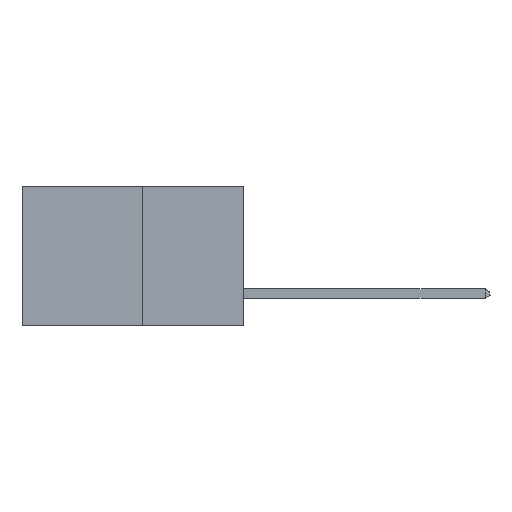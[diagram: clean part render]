
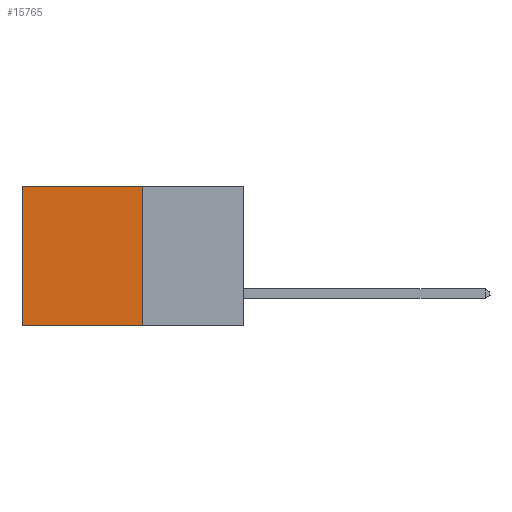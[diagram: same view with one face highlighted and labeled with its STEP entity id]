
A CAD part, left-side view. The second image highlights one B-rep face of the part: STEP entity #15765.
In plain terms, the highlighted planar face has unit normal (-1, 0, 0).
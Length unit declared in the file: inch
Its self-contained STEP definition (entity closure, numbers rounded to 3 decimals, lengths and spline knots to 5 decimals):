
#330 = ORIENTED_EDGE ( 'NONE', *, *, #22744, .F. ) ;
#1089 = FACE_OUTER_BOUND ( 'NONE', #14952, .T. ) ;
#1343 = CARTESIAN_POINT ( 'NONE',  ( 0.277, 0.59, 0. ) ) ;
#2663 = VERTEX_POINT ( 'NONE', #25997 ) ;
#2810 = VERTEX_POINT ( 'NONE', #24809 ) ;
#4584 = CARTESIAN_POINT ( 'NONE',  ( 0.277, 0.59, -0.37 ) ) ;
#5009 = EDGE_CURVE ( 'NONE', #7371, #24351, #25467, .T. ) ;
#5277 = DIRECTION ( 'NONE',  ( 0., 0., -1. ) ) ;
#5371 = VECTOR ( 'NONE', #13319, 39.37008 ) ;
#5884 = DIRECTION ( 'NONE',  ( 0., 1., 0. ) ) ;
#6925 = DIRECTION ( 'NONE',  ( 0., 0., -1. ) ) ;
#7193 = CARTESIAN_POINT ( 'NONE',  ( 0.277, 0.27, -0.37 ) ) ;
#7371 = VERTEX_POINT ( 'NONE', #1343 ) ;
#8189 = CARTESIAN_POINT ( 'NONE',  ( 0.277, 0.59, -0.37 ) ) ;
#9144 = ORIENTED_EDGE ( 'NONE', *, *, #20478, .F. ) ;
#10386 = DIRECTION ( 'NONE',  ( 0., 0., -1. ) ) ;
#13319 = DIRECTION ( 'NONE',  ( 0., 1., 0. ) ) ;
#13641 = AXIS2_PLACEMENT_3D ( 'NONE', #14484, #22718, #10386 ) ;
#13699 = LINE ( 'NONE', #16180, #24578 ) ;
#14484 = CARTESIAN_POINT ( 'NONE',  ( 0.277, 0.27, -0.37 ) ) ;
#14658 = VECTOR ( 'NONE', #5277, 39.37008 ) ;
#14952 = EDGE_LOOP ( 'NONE', ( #18817, #330, #9144, #19706 ) ) ;
#15719 = LINE ( 'NONE', #7193, #5371 ) ;
#15765 = ADVANCED_FACE ( 'NONE', ( #1089 ), #18647, .F. ) ;
#16180 = CARTESIAN_POINT ( 'NONE',  ( 0.277, 0.27, 0. ) ) ;
#18647 = PLANE ( 'NONE',  #13641 ) ;
#18817 = ORIENTED_EDGE ( 'NONE', *, *, #5009, .T. ) ;
#19320 = CARTESIAN_POINT ( 'NONE',  ( 0.277, 0.27, -0.37 ) ) ;
#19706 = ORIENTED_EDGE ( 'NONE', *, *, #23641, .T. ) ;
#20478 = EDGE_CURVE ( 'NONE', #2810, #2663, #20657, .T. ) ;
#20657 = LINE ( 'NONE', #19320, #25977 ) ;
#22718 = DIRECTION ( 'NONE',  ( 1., 0., 0. ) ) ;
#22744 = EDGE_CURVE ( 'NONE', #2663, #24351, #15719, .T. ) ;
#23641 = EDGE_CURVE ( 'NONE', #2810, #7371, #13699, .T. ) ;
#24351 = VERTEX_POINT ( 'NONE', #8189 ) ;
#24578 = VECTOR ( 'NONE', #5884, 39.37008 ) ;
#24809 = CARTESIAN_POINT ( 'NONE',  ( 0.277, 0.27, 0. ) ) ;
#25467 = LINE ( 'NONE', #4584, #14658 ) ;
#25977 = VECTOR ( 'NONE', #6925, 39.37008 ) ;
#25997 = CARTESIAN_POINT ( 'NONE',  ( 0.277, 0.27, -0.37 ) ) ;
